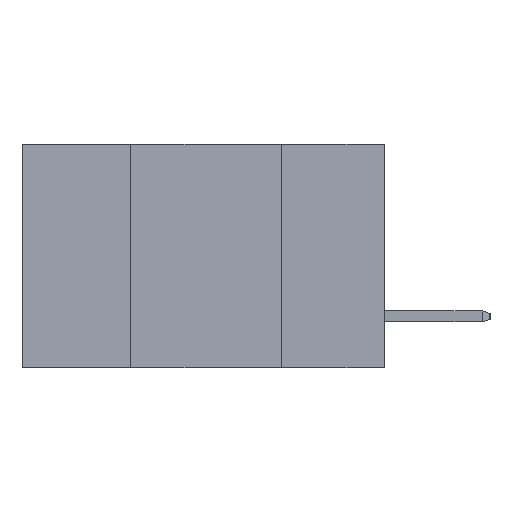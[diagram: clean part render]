
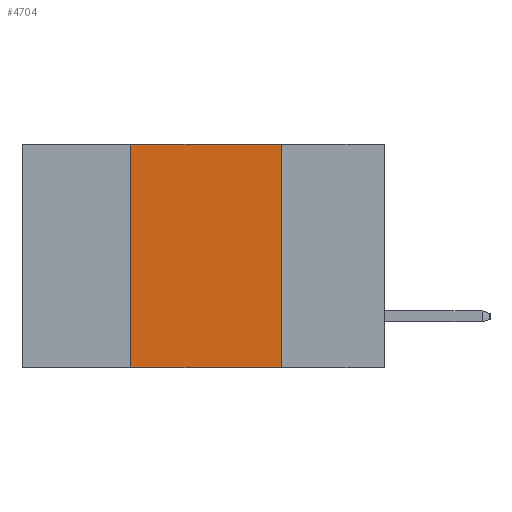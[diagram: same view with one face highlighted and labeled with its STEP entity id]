
A CAD part, left-side view. The second image highlights one B-rep face of the part: STEP entity #4704.
In plain terms, the highlighted planar face has unit normal (-1, 0, 0).
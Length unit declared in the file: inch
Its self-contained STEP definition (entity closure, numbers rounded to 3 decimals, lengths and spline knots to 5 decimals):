
#393 = EDGE_CURVE ( 'NONE', #16837, #2573, #10741, .T. ) ;
#861 = VERTEX_POINT ( 'NONE', #7972 ) ;
#1335 = CARTESIAN_POINT ( 'NONE',  ( 0., 0.17, 0. ) ) ;
#1929 = CARTESIAN_POINT ( 'NONE',  ( 0., 0.6, -0.37 ) ) ;
#2573 = VERTEX_POINT ( 'NONE', #1335 ) ;
#2684 = EDGE_LOOP ( 'NONE', ( #5188, #16960, #3655, #4538 ) ) ;
#2917 = VECTOR ( 'NONE', #7509, 39.37008 ) ;
#3655 = ORIENTED_EDGE ( 'NONE', *, *, #17874, .F. ) ;
#4538 = ORIENTED_EDGE ( 'NONE', *, *, #10190, .T. ) ;
#4704 = ADVANCED_FACE ( 'NONE', ( #12468 ), #6207, .F. ) ;
#5188 = ORIENTED_EDGE ( 'NONE', *, *, #7025, .F. ) ;
#5675 = VECTOR ( 'NONE', #17180, 39.37008 ) ;
#6207 = PLANE ( 'NONE',  #8925 ) ;
#7025 = EDGE_CURVE ( 'NONE', #2573, #7713, #14740, .T. ) ;
#7232 = CARTESIAN_POINT ( 'NONE',  ( 0., 0.17, -0.37 ) ) ;
#7447 = LINE ( 'NONE', #7652, #14539 ) ;
#7509 = DIRECTION ( 'NONE',  ( 0., -1., 0. ) ) ;
#7613 = DIRECTION ( 'NONE',  ( 0., 0., -1. ) ) ;
#7652 = CARTESIAN_POINT ( 'NONE',  ( 0., 0.42, -0.37 ) ) ;
#7713 = VERTEX_POINT ( 'NONE', #8924 ) ;
#7972 = CARTESIAN_POINT ( 'NONE',  ( 0., 0.42, -0.37 ) ) ;
#8924 = CARTESIAN_POINT ( 'NONE',  ( 0., 0.17, -0.37 ) ) ;
#8925 = AXIS2_PLACEMENT_3D ( 'NONE', #8956, #16113, #7613 ) ;
#8956 = CARTESIAN_POINT ( 'NONE',  ( 0., 0.6, 0. ) ) ;
#10190 = EDGE_CURVE ( 'NONE', #861, #7713, #10827, .T. ) ;
#10465 = DIRECTION ( 'NONE',  ( 0., 0., 1. ) ) ;
#10741 = LINE ( 'NONE', #11261, #17919 ) ;
#10827 = LINE ( 'NONE', #1929, #2917 ) ;
#11261 = CARTESIAN_POINT ( 'NONE',  ( 0., 0.6, 0. ) ) ;
#12468 = FACE_OUTER_BOUND ( 'NONE', #2684, .T. ) ;
#12483 = CARTESIAN_POINT ( 'NONE',  ( 0., 0.42, 0. ) ) ;
#14539 = VECTOR ( 'NONE', #10465, 39.37008 ) ;
#14740 = LINE ( 'NONE', #7232, #5675 ) ;
#16113 = DIRECTION ( 'NONE',  ( 1., 0., 0. ) ) ;
#16214 = DIRECTION ( 'NONE',  ( 0., -1., 0. ) ) ;
#16837 = VERTEX_POINT ( 'NONE', #12483 ) ;
#16960 = ORIENTED_EDGE ( 'NONE', *, *, #393, .F. ) ;
#17180 = DIRECTION ( 'NONE',  ( 0., 0., -1. ) ) ;
#17874 = EDGE_CURVE ( 'NONE', #861, #16837, #7447, .T. ) ;
#17919 = VECTOR ( 'NONE', #16214, 39.37008 ) ;
